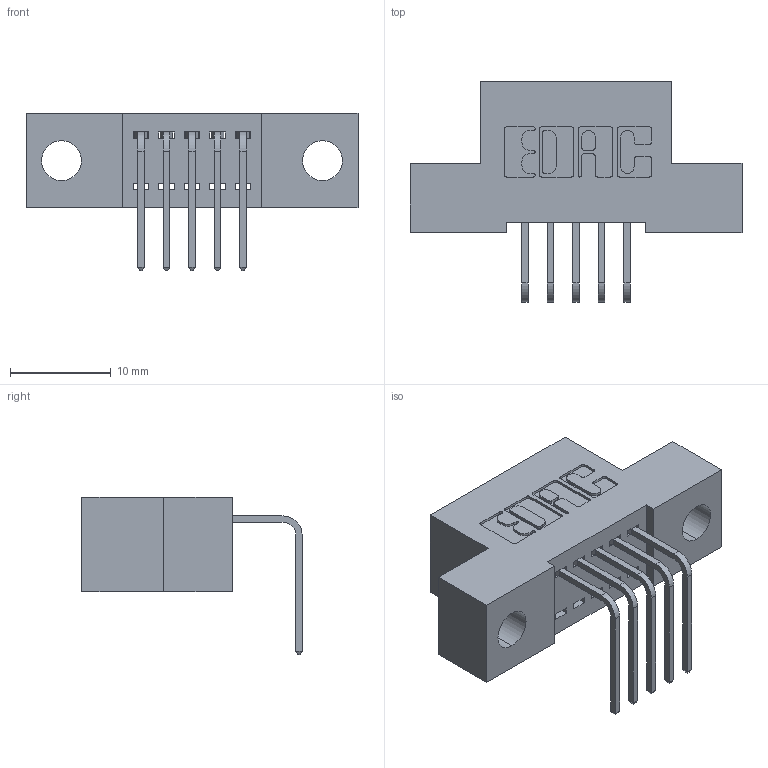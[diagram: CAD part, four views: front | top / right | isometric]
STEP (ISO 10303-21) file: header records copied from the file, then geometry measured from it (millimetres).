
FILE_DESCRIPTION (( 'STEP AP203' ), '1' );
FILE_NAME ('392-005-558-104.STEP', '2018-08-14T17:22:53', ( '' ), ( '' ), 'SwSTEP 2.0', 'SolidWorks 2016', '' );
FILE_SCHEMA (( 'CONFIG_CONTROL_DESIGN' ));
Length unit declared in the file: inch
Products named in the file (3): 342 Part_.156 TH; 345-292-001_558 Tail - 2; 392-005-558-104
Assembly tree (6 placements, depth 2):
  392-005-558-104
    342 Part_.156 TH
    345-292-001_558 Tail - 2  x5
Bounding box: 33.02 x 21.91 x 15.62 mm (x, y, z)
Volume: 2688.5 mm3; surface area: 3170.6 mm2
Topology: 6 solids, 6 shells, 410 faces, 1209 edges, 798 vertices
Faces by surface type: plane 286, cylinder 124
Entity records: 7797 total; most frequent: CARTESIAN_POINT 1357, ORIENTED_EDGE 1298, DIRECTION 1219, EDGE_CURVE 649, LINE 521, VECTOR 521, VERTEX_POINT 430, AXIS2_PLACEMENT_3D 349
